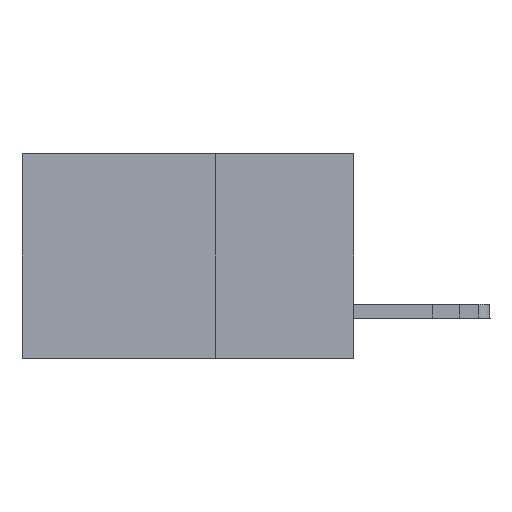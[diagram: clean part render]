
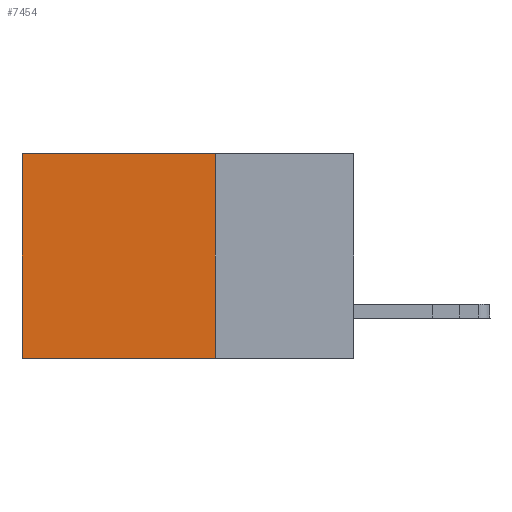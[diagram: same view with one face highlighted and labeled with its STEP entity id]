
A CAD part, left-side view. The second image highlights one B-rep face of the part: STEP entity #7454.
In plain terms, the highlighted planar face has unit normal (-1, 0, 0).
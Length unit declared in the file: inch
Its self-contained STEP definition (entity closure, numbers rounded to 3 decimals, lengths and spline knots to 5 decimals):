
#1602 = CARTESIAN_POINT ( 'NONE',  ( 0.2875, 0.25, 0. ) ) ;
#1768 = VERTEX_POINT ( 'NONE', #7806 ) ;
#1835 = CARTESIAN_POINT ( 'NONE',  ( 0.2875, 0.6, 0. ) ) ;
#2037 = CARTESIAN_POINT ( 'NONE',  ( 0.2875, 0.25, 0. ) ) ;
#2285 = DIRECTION ( 'NONE',  ( 0., 1., 0. ) ) ;
#2505 = AXIS2_PLACEMENT_3D ( 'NONE', #1602, #4580, #14918 ) ;
#2697 = VECTOR ( 'NONE', #5024, 39.37008 ) ;
#3098 = PLANE ( 'NONE',  #2505 ) ;
#3641 = FACE_OUTER_BOUND ( 'NONE', #9502, .T. ) ;
#3844 = VECTOR ( 'NONE', #12280, 39.37008 ) ;
#3985 = ORIENTED_EDGE ( 'NONE', *, *, #16646, .T. ) ;
#4291 = VECTOR ( 'NONE', #7846, 39.37008 ) ;
#4580 = DIRECTION ( 'NONE',  ( 1., 0., 0. ) ) ;
#4888 = CARTESIAN_POINT ( 'NONE',  ( 0.2875, 0.25, 0. ) ) ;
#4918 = EDGE_CURVE ( 'NONE', #17797, #1768, #14423, .T. ) ;
#5024 = DIRECTION ( 'NONE',  ( 0., 1., 0. ) ) ;
#5431 = ORIENTED_EDGE ( 'NONE', *, *, #9054, .T. ) ;
#7454 = ADVANCED_FACE ( 'NONE', ( #3641 ), #3098, .F. ) ;
#7806 = CARTESIAN_POINT ( 'NONE',  ( 0.2875, 0.6, -0.37 ) ) ;
#7846 = DIRECTION ( 'NONE',  ( 0., 0., -1. ) ) ;
#8145 = EDGE_CURVE ( 'NONE', #15535, #17797, #15643, .T. ) ;
#9054 = EDGE_CURVE ( 'NONE', #15535, #12445, #10293, .T. ) ;
#9177 = LINE ( 'NONE', #1835, #4291 ) ;
#9502 = EDGE_LOOP ( 'NONE', ( #3985, #15688, #13914, #5431 ) ) ;
#10293 = LINE ( 'NONE', #2037, #2697 ) ;
#12059 = CARTESIAN_POINT ( 'NONE',  ( 0.2875, 0.25, -0.37 ) ) ;
#12280 = DIRECTION ( 'NONE',  ( 0., 0., -1. ) ) ;
#12445 = VERTEX_POINT ( 'NONE', #16927 ) ;
#13740 = CARTESIAN_POINT ( 'NONE',  ( 0.2875, 0.25, 0. ) ) ;
#13914 = ORIENTED_EDGE ( 'NONE', *, *, #8145, .F. ) ;
#13950 = VECTOR ( 'NONE', #2285, 39.37008 ) ;
#14079 = CARTESIAN_POINT ( 'NONE',  ( 0.2875, 0.25, -0.37 ) ) ;
#14423 = LINE ( 'NONE', #14079, #13950 ) ;
#14918 = DIRECTION ( 'NONE',  ( 0., 0., -1. ) ) ;
#15535 = VERTEX_POINT ( 'NONE', #13740 ) ;
#15643 = LINE ( 'NONE', #4888, #3844 ) ;
#15688 = ORIENTED_EDGE ( 'NONE', *, *, #4918, .F. ) ;
#16646 = EDGE_CURVE ( 'NONE', #12445, #1768, #9177, .T. ) ;
#16927 = CARTESIAN_POINT ( 'NONE',  ( 0.2875, 0.6, 0. ) ) ;
#17797 = VERTEX_POINT ( 'NONE', #12059 ) ;
